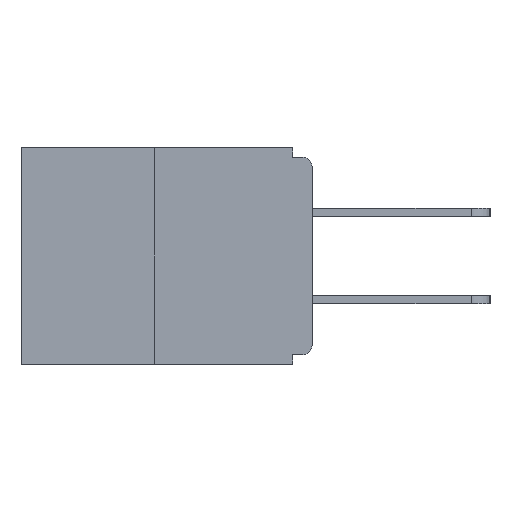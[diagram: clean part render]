
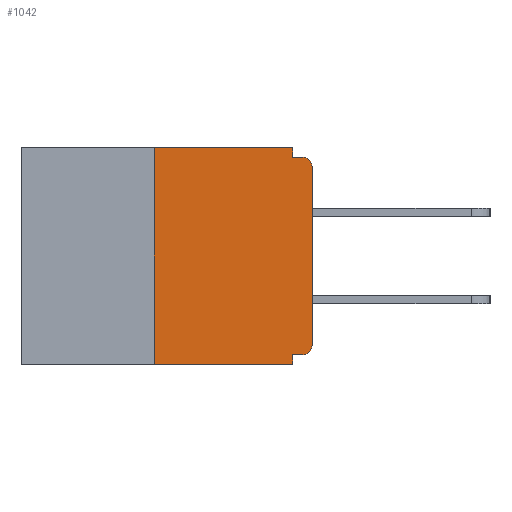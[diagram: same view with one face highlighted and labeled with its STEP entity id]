
A CAD part, left-side view. The second image highlights one B-rep face of the part: STEP entity #1042.
In plain terms, the highlighted planar face has unit normal (-1, 0, 0).
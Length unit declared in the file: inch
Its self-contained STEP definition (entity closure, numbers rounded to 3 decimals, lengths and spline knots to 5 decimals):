
#101 = ORIENTED_EDGE ( 'NONE', *, *, #6887, .F. ) ;
#652 = VERTEX_POINT ( 'NONE', #11440 ) ;
#837 = DIRECTION ( 'NONE',  ( 0., -1., 0. ) ) ;
#845 = EDGE_CURVE ( 'NONE', #6285, #13045, #2315, .T. ) ;
#949 = FACE_OUTER_BOUND ( 'NONE', #4262, .T. ) ;
#1042 = ADVANCED_FACE ( 'NONE', ( #949 ), #4895, .F. ) ;
#1243 = LINE ( 'NONE', #5376, #1556 ) ;
#1277 = ORIENTED_EDGE ( 'NONE', *, *, #11212, .F. ) ;
#1500 = VERTEX_POINT ( 'NONE', #6486 ) ;
#1556 = VECTOR ( 'NONE', #11634, 39.37008 ) ;
#1974 = ORIENTED_EDGE ( 'NONE', *, *, #4396, .T. ) ;
#2170 = VERTEX_POINT ( 'NONE', #12763 ) ;
#2306 = CARTESIAN_POINT ( 'NONE',  ( 0., 0.015, -0.328 ) ) ;
#2315 = LINE ( 'NONE', #6373, #8153 ) ;
#2480 = CARTESIAN_POINT ( 'NONE',  ( 0., 0.031, 0. ) ) ;
#2550 = EDGE_CURVE ( 'NONE', #13045, #3830, #11417, .T. ) ;
#2617 = CARTESIAN_POINT ( 'NONE',  ( 0., 0.015, -0.313 ) ) ;
#2758 = ORIENTED_EDGE ( 'NONE', *, *, #3088, .F. ) ;
#2848 = CARTESIAN_POINT ( 'NONE',  ( 0., 0.46, -0.343 ) ) ;
#2862 = LINE ( 'NONE', #11317, #7705 ) ;
#2868 = VECTOR ( 'NONE', #6214, 39.37008 ) ;
#3088 = EDGE_CURVE ( 'NONE', #3830, #3940, #10130, .T. ) ;
#3644 = DIRECTION ( 'NONE',  ( -1., 0., 0. ) ) ;
#3830 = VERTEX_POINT ( 'NONE', #2480 ) ;
#3893 = CARTESIAN_POINT ( 'NONE',  ( 0., 0.46, 0. ) ) ;
#3940 = VERTEX_POINT ( 'NONE', #5797 ) ;
#4262 = EDGE_LOOP ( 'NONE', ( #8515, #8341, #7879, #1277, #101, #6743, #12037, #1974, #7964, #2758 ) ) ;
#4396 = EDGE_CURVE ( 'NONE', #2170, #12601, #4399, .T. ) ;
#4399 = CIRCLE ( 'NONE', #11904, 0.015 ) ;
#4636 = EDGE_CURVE ( 'NONE', #3940, #12601, #1243, .T. ) ;
#4895 = PLANE ( 'NONE',  #13040 ) ;
#5376 = CARTESIAN_POINT ( 'NONE',  ( 0., 0., -0.015 ) ) ;
#5549 = AXIS2_PLACEMENT_3D ( 'NONE', #2617, #11936, #6808 ) ;
#5797 = CARTESIAN_POINT ( 'NONE',  ( 0., 0.031, -0.015 ) ) ;
#6069 = LINE ( 'NONE', #8093, #6680 ) ;
#6214 = DIRECTION ( 'NONE',  ( 0., -1., 0. ) ) ;
#6285 = VERTEX_POINT ( 'NONE', #7871 ) ;
#6290 = VECTOR ( 'NONE', #837, 39.37008 ) ;
#6373 = CARTESIAN_POINT ( 'NONE',  ( 0., 0.25, 0. ) ) ;
#6486 = CARTESIAN_POINT ( 'NONE',  ( 0., 0., -0.313 ) ) ;
#6680 = VECTOR ( 'NONE', #13260, 39.37008 ) ;
#6722 = CARTESIAN_POINT ( 'NONE',  ( 0., 0.015, -0.03 ) ) ;
#6743 = ORIENTED_EDGE ( 'NONE', *, *, #12020, .T. ) ;
#6808 = DIRECTION ( 'NONE',  ( 0., 0., -1. ) ) ;
#6887 = EDGE_CURVE ( 'NONE', #8946, #10084, #6069, .T. ) ;
#6896 = DIRECTION ( 'NONE',  ( 0., 0., -1. ) ) ;
#7269 = CIRCLE ( 'NONE', #5549, 0.015 ) ;
#7705 = VECTOR ( 'NONE', #9150, 39.37008 ) ;
#7808 = DIRECTION ( 'NONE',  ( 0., 0., -1. ) ) ;
#7871 = CARTESIAN_POINT ( 'NONE',  ( 0., 0.25, -0.343 ) ) ;
#7879 = ORIENTED_EDGE ( 'NONE', *, *, #8640, .T. ) ;
#7964 = ORIENTED_EDGE ( 'NONE', *, *, #4636, .F. ) ;
#8093 = CARTESIAN_POINT ( 'NONE',  ( 0., 0., -0.328 ) ) ;
#8153 = VECTOR ( 'NONE', #10481, 39.37008 ) ;
#8341 = ORIENTED_EDGE ( 'NONE', *, *, #845, .F. ) ;
#8515 = ORIENTED_EDGE ( 'NONE', *, *, #2550, .F. ) ;
#8640 = EDGE_CURVE ( 'NONE', #6285, #652, #12026, .T. ) ;
#8863 = LINE ( 'NONE', #10738, #13200 ) ;
#8946 = VERTEX_POINT ( 'NONE', #2306 ) ;
#9125 = DIRECTION ( 'NONE',  ( 0., 0., -1. ) ) ;
#9150 = DIRECTION ( 'NONE',  ( 0., 0., -1. ) ) ;
#9306 = VECTOR ( 'NONE', #9125, 39.37008 ) ;
#9938 = DIRECTION ( 'NONE',  ( 1., 0., 0. ) ) ;
#10084 = VERTEX_POINT ( 'NONE', #11765 ) ;
#10130 = LINE ( 'NONE', #11094, #9306 ) ;
#10481 = DIRECTION ( 'NONE',  ( 0., 0., 1. ) ) ;
#10656 = EDGE_CURVE ( 'NONE', #1500, #2170, #8863, .T. ) ;
#10738 = CARTESIAN_POINT ( 'NONE',  ( 0., 0., 0. ) ) ;
#11094 = CARTESIAN_POINT ( 'NONE',  ( 0., 0.031, 0. ) ) ;
#11115 = CARTESIAN_POINT ( 'NONE',  ( 0., 0.015, -0.015 ) ) ;
#11212 = EDGE_CURVE ( 'NONE', #10084, #652, #2862, .T. ) ;
#11317 = CARTESIAN_POINT ( 'NONE',  ( 0., 0.031, -0.343 ) ) ;
#11365 = CARTESIAN_POINT ( 'NONE',  ( 0., 0.25, 0. ) ) ;
#11417 = LINE ( 'NONE', #12420, #2868 ) ;
#11440 = CARTESIAN_POINT ( 'NONE',  ( 0., 0.031, -0.343 ) ) ;
#11634 = DIRECTION ( 'NONE',  ( 0., -1., 0. ) ) ;
#11765 = CARTESIAN_POINT ( 'NONE',  ( 0., 0.031, -0.328 ) ) ;
#11904 = AXIS2_PLACEMENT_3D ( 'NONE', #6722, #3644, #7808 ) ;
#11936 = DIRECTION ( 'NONE',  ( -1., 0., 0. ) ) ;
#12020 = EDGE_CURVE ( 'NONE', #8946, #1500, #7269, .T. ) ;
#12026 = LINE ( 'NONE', #2848, #6290 ) ;
#12037 = ORIENTED_EDGE ( 'NONE', *, *, #10656, .T. ) ;
#12420 = CARTESIAN_POINT ( 'NONE',  ( 0., 0.46, 0. ) ) ;
#12601 = VERTEX_POINT ( 'NONE', #11115 ) ;
#12763 = CARTESIAN_POINT ( 'NONE',  ( 0., 0., -0.03 ) ) ;
#12970 = DIRECTION ( 'NONE',  ( 0., 0., 1. ) ) ;
#13040 = AXIS2_PLACEMENT_3D ( 'NONE', #3893, #9938, #6896 ) ;
#13045 = VERTEX_POINT ( 'NONE', #11365 ) ;
#13200 = VECTOR ( 'NONE', #12970, 39.37008 ) ;
#13260 = DIRECTION ( 'NONE',  ( 0., 1., 0. ) ) ;
